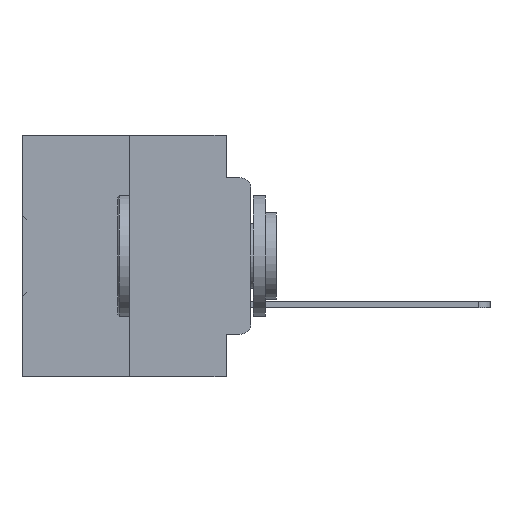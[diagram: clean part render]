
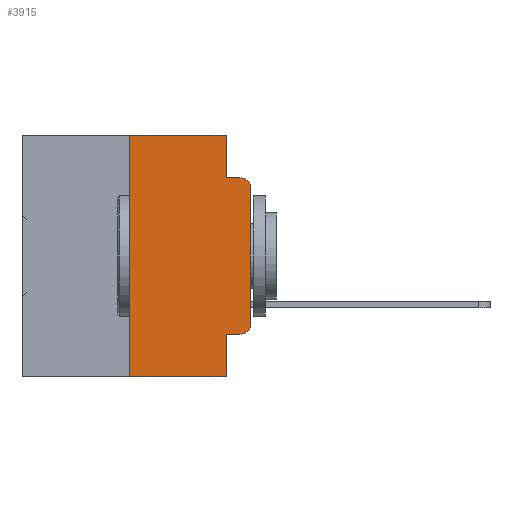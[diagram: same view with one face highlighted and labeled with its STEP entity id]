
A CAD part, left-side view. The second image highlights one B-rep face of the part: STEP entity #3915.
In plain terms, the highlighted planar face has unit normal (-1, 0, 0).
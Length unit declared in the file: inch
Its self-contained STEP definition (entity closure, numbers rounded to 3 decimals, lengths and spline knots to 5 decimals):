
#34 = EDGE_CURVE ( 'NONE', #36807, #2840, #9313, .T. ) ;
#281 = DIRECTION ( 'NONE',  ( 0., 0., 1. ) ) ;
#587 = VERTEX_POINT ( 'NONE', #16509 ) ;
#1196 = CARTESIAN_POINT ( 'NONE',  ( 0., 0.25, 0. ) ) ;
#1586 = ORIENTED_EDGE ( 'NONE', *, *, #3386, .F. ) ;
#2521 = VECTOR ( 'NONE', #14019, 39.37008 ) ;
#2781 = DIRECTION ( 'NONE',  ( 0., 0., -1. ) ) ;
#2840 = VERTEX_POINT ( 'NONE', #33712 ) ;
#3386 = EDGE_CURVE ( 'NONE', #23904, #9069, #32339, .T. ) ;
#3461 = CARTESIAN_POINT ( 'NONE',  ( 0., 0., -0.1085 ) ) ;
#3834 = CARTESIAN_POINT ( 'NONE',  ( 0., 0.02, -0.1085 ) ) ;
#3915 = ADVANCED_FACE ( 'NONE', ( #19340 ), #35139, .F. ) ;
#4290 = CARTESIAN_POINT ( 'NONE',  ( 0., 0.051, -0.0885 ) ) ;
#4611 = DIRECTION ( 'NONE',  ( 0., 0., -1. ) ) ;
#4734 = EDGE_CURVE ( 'NONE', #587, #23865, #34527, .T. ) ;
#4811 = CARTESIAN_POINT ( 'NONE',  ( 0., 0.051, 0. ) ) ;
#6135 = ORIENTED_EDGE ( 'NONE', *, *, #7639, .T. ) ;
#7109 = DIRECTION ( 'NONE',  ( 0., 0., -1. ) ) ;
#7639 = EDGE_CURVE ( 'NONE', #2840, #9490, #33094, .T. ) ;
#7889 = CARTESIAN_POINT ( 'NONE',  ( 0., 0.051, -0.4115 ) ) ;
#8206 = DIRECTION ( 'NONE',  ( 0., -1., 0. ) ) ;
#8229 = VERTEX_POINT ( 'NONE', #29726 ) ;
#8265 = ORIENTED_EDGE ( 'NONE', *, *, #19718, .F. ) ;
#9069 = VERTEX_POINT ( 'NONE', #4811 ) ;
#9189 = EDGE_CURVE ( 'NONE', #27203, #36807, #10200, .T. ) ;
#9313 = CIRCLE ( 'NONE', #20657, 0.02 ) ;
#9490 = VERTEX_POINT ( 'NONE', #3461 ) ;
#9927 = VECTOR ( 'NONE', #37178, 39.37008 ) ;
#10200 = LINE ( 'NONE', #38040, #21410 ) ;
#10247 = DIRECTION ( 'NONE',  ( 0., -1., 0. ) ) ;
#10739 = ORIENTED_EDGE ( 'NONE', *, *, #24918, .F. ) ;
#11579 = CARTESIAN_POINT ( 'NONE',  ( 0., 0.25, 0. ) ) ;
#12403 = CARTESIAN_POINT ( 'NONE',  ( 0., 0.051, -0.0885 ) ) ;
#12704 = VECTOR ( 'NONE', #10247, 39.37008 ) ;
#13480 = VECTOR ( 'NONE', #4611, 39.37008 ) ;
#14019 = DIRECTION ( 'NONE',  ( 0., 0., -1. ) ) ;
#15027 = ORIENTED_EDGE ( 'NONE', *, *, #35050, .F. ) ;
#16125 = DIRECTION ( 'NONE',  ( -1., 0., 0. ) ) ;
#16234 = AXIS2_PLACEMENT_3D ( 'NONE', #3834, #16125, #7109 ) ;
#16509 = CARTESIAN_POINT ( 'NONE',  ( 0., 0.25, -0.5 ) ) ;
#17252 = ORIENTED_EDGE ( 'NONE', *, *, #33791, .F. ) ;
#19014 = CARTESIAN_POINT ( 'NONE',  ( 0., 0.473, -0.5 ) ) ;
#19340 = FACE_OUTER_BOUND ( 'NONE', #26143, .T. ) ;
#19353 = CARTESIAN_POINT ( 'NONE',  ( 0., 0.051, 0. ) ) ;
#19473 = VECTOR ( 'NONE', #26850, 39.37008 ) ;
#19718 = EDGE_CURVE ( 'NONE', #25398, #8229, #27327, .T. ) ;
#20633 = CARTESIAN_POINT ( 'NONE',  ( 0., 0.473, 0. ) ) ;
#20657 = AXIS2_PLACEMENT_3D ( 'NONE', #37175, #25396, #31487 ) ;
#21372 = LINE ( 'NONE', #19353, #13480 ) ;
#21410 = VECTOR ( 'NONE', #8206, 39.37008 ) ;
#22530 = CARTESIAN_POINT ( 'NONE',  ( 0., 0.051, -0.5 ) ) ;
#23865 = VERTEX_POINT ( 'NONE', #22530 ) ;
#23904 = VERTEX_POINT ( 'NONE', #11579 ) ;
#24148 = DIRECTION ( 'NONE',  ( 0., -1., 0. ) ) ;
#24918 = EDGE_CURVE ( 'NONE', #27203, #23865, #21372, .T. ) ;
#25396 = DIRECTION ( 'NONE',  ( -1., 0., 0. ) ) ;
#25398 = VERTEX_POINT ( 'NONE', #4290 ) ;
#26143 = EDGE_LOOP ( 'NONE', ( #6135, #28047, #8265, #17252, #1586, #15027, #28156, #10739, #31089, #26821 ) ) ;
#26821 = ORIENTED_EDGE ( 'NONE', *, *, #34, .T. ) ;
#26850 = DIRECTION ( 'NONE',  ( 0., -1., 0. ) ) ;
#27203 = VERTEX_POINT ( 'NONE', #7889 ) ;
#27327 = LINE ( 'NONE', #12403, #19473 ) ;
#28047 = ORIENTED_EDGE ( 'NONE', *, *, #30971, .T. ) ;
#28156 = ORIENTED_EDGE ( 'NONE', *, *, #4734, .T. ) ;
#28167 = VECTOR ( 'NONE', #24148, 39.37008 ) ;
#29090 = LINE ( 'NONE', #31658, #2521 ) ;
#29431 = AXIS2_PLACEMENT_3D ( 'NONE', #20633, #35388, #2781 ) ;
#29726 = CARTESIAN_POINT ( 'NONE',  ( 0., 0.02, -0.0885 ) ) ;
#30971 = EDGE_CURVE ( 'NONE', #9490, #8229, #35783, .T. ) ;
#31089 = ORIENTED_EDGE ( 'NONE', *, *, #9189, .T. ) ;
#31343 = LINE ( 'NONE', #1196, #9927 ) ;
#31487 = DIRECTION ( 'NONE',  ( 0., 0., -1. ) ) ;
#31658 = CARTESIAN_POINT ( 'NONE',  ( 0., 0.051, 0. ) ) ;
#31731 = VECTOR ( 'NONE', #281, 39.37008 ) ;
#32339 = LINE ( 'NONE', #33336, #28167 ) ;
#33094 = LINE ( 'NONE', #36166, #31731 ) ;
#33336 = CARTESIAN_POINT ( 'NONE',  ( 0., 0.473, 0. ) ) ;
#33712 = CARTESIAN_POINT ( 'NONE',  ( 0., 0., -0.3915 ) ) ;
#33791 = EDGE_CURVE ( 'NONE', #9069, #25398, #29090, .T. ) ;
#34527 = LINE ( 'NONE', #19014, #12704 ) ;
#35050 = EDGE_CURVE ( 'NONE', #587, #23904, #31343, .T. ) ;
#35139 = PLANE ( 'NONE',  #29431 ) ;
#35388 = DIRECTION ( 'NONE',  ( 1., 0., 0. ) ) ;
#35783 = CIRCLE ( 'NONE', #16234, 0.02 ) ;
#36166 = CARTESIAN_POINT ( 'NONE',  ( 0., 0., 0. ) ) ;
#36795 = CARTESIAN_POINT ( 'NONE',  ( 0., 0.02, -0.4115 ) ) ;
#36807 = VERTEX_POINT ( 'NONE', #36795 ) ;
#37175 = CARTESIAN_POINT ( 'NONE',  ( 0., 0.02, -0.3915 ) ) ;
#37178 = DIRECTION ( 'NONE',  ( 0., 0., 1. ) ) ;
#38040 = CARTESIAN_POINT ( 'NONE',  ( 0., 0.051, -0.4115 ) ) ;
